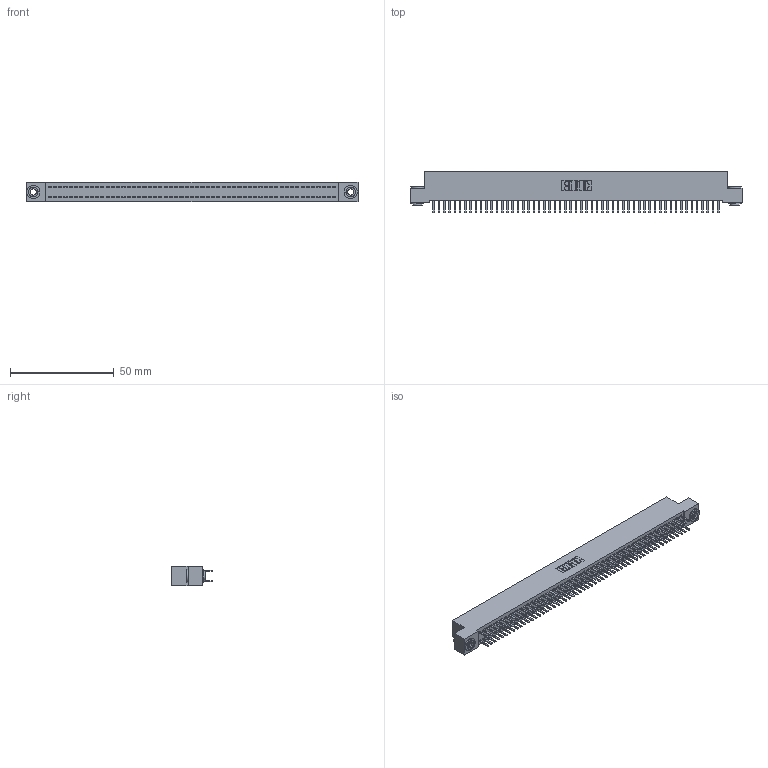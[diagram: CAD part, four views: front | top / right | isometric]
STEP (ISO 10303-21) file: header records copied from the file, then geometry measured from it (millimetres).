
FILE_DESCRIPTION (( 'STEP AP203' ), '1' );
FILE_NAME ('342-110-520-203.STEP', '2018-08-14T11:18:16', ( '' ), ( '' ), 'SwSTEP 2.0', 'SolidWorks 2016', '' );
FILE_SCHEMA (( 'CONFIG_CONTROL_DESIGN' ));
Length unit declared in the file: inch
Products named in the file (4): 342-250-002_345-250-002-102; 342-110-520-203; 342 Part_.156 TH; 345-292-001_345-293-120
Assembly tree (113 placements, depth 2):
  342-110-520-203
    342 Part_.156 TH
    345-292-001_345-293-120  x110
    342-250-002_345-250-002-102  x2
Bounding box: 160.02 x 20.02 x 9.4 mm (x, y, z)
Volume: 14413.8 mm3; surface area: 23882.3 mm2
Topology: 113 solids, 113 shells, 6308 faces, 18305 edges, 11906 vertices
Faces by surface type: plane 4256, cylinder 2044, cone 8
Entity records: 34334 total; most frequent: CARTESIAN_POINT 5661, ORIENTED_EDGE 5578, DIRECTION 4835, EDGE_CURVE 2789, VECTOR 2633, LINE 2633, VERTEX_POINT 1854, AXIS2_PLACEMENT_3D 1101
